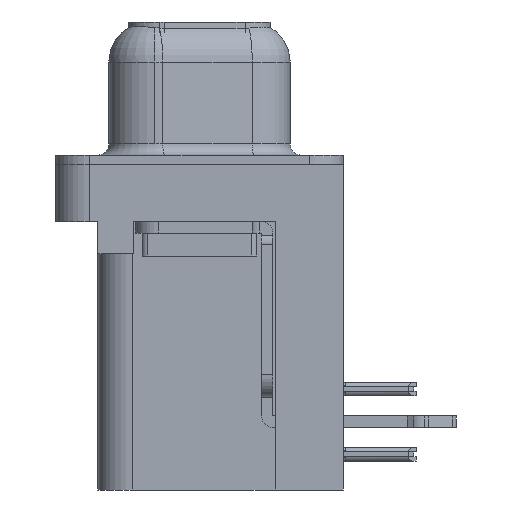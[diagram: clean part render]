
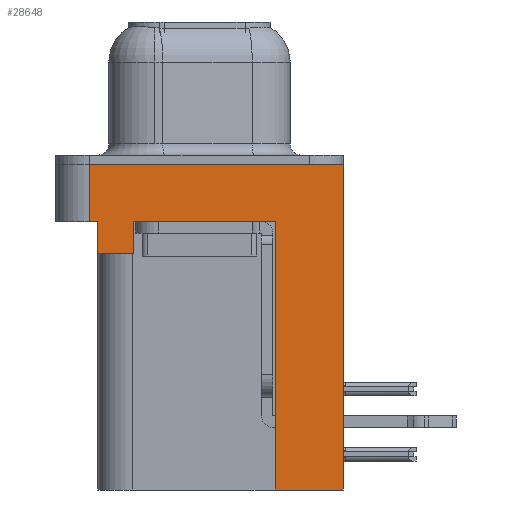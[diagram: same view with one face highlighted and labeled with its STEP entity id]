
A CAD part, left-side view. The second image highlights one B-rep face of the part: STEP entity #28648.
In plain terms, the highlighted planar face has unit normal (-1, 0, 0).
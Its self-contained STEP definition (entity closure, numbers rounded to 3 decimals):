
#189 = CARTESIAN_POINT ( 'NONE',  ( -2.91, 4.425, -3.9 ) ) ;
#225 = EDGE_CURVE ( 'NONE', #4165, #5498, #7820, .T. ) ;
#361 = CARTESIAN_POINT ( 'NONE',  ( -2.91, -6.275, 0. ) ) ;
#401 = LINE ( 'NONE', #21651, #32084 ) ;
#633 = EDGE_CURVE ( 'NONE', #26346, #26637, #401, .T. ) ;
#636 = EDGE_CURVE ( 'NONE', #27054, #9915, #24114, .T. ) ;
#830 = CARTESIAN_POINT ( 'NONE',  ( -2.91, -3.295, -14.2 ) ) ;
#1801 = ORIENTED_EDGE ( 'NONE', *, *, #12141, .F. ) ;
#2073 = CARTESIAN_POINT ( 'NONE',  ( -2.91, 2.895, -2.5 ) ) ;
#3632 = FACE_OUTER_BOUND ( 'NONE', #15709, .T. ) ;
#3735 = CARTESIAN_POINT ( 'NONE',  ( -2.91, 4.775, -2.5 ) ) ;
#4165 = VERTEX_POINT ( 'NONE', #10867 ) ;
#4537 = DIRECTION ( 'NONE',  ( 0., 0., 1. ) ) ;
#4563 = AXIS2_PLACEMENT_3D ( 'NONE', #25066, #22414, #33117 ) ;
#5385 = ORIENTED_EDGE ( 'NONE', *, *, #12654, .F. ) ;
#5498 = VERTEX_POINT ( 'NONE', #2073 ) ;
#5653 = VECTOR ( 'NONE', #29345, 1000. ) ;
#6954 = DIRECTION ( 'NONE',  ( 0., -1., 0. ) ) ;
#7522 = LINE ( 'NONE', #31911, #12522 ) ;
#7767 = VECTOR ( 'NONE', #19387, 1000. ) ;
#7820 = LINE ( 'NONE', #29422, #11222 ) ;
#9086 = VECTOR ( 'NONE', #6954, 1000. ) ;
#9915 = VERTEX_POINT ( 'NONE', #27889 ) ;
#10867 = CARTESIAN_POINT ( 'NONE',  ( -2.91, 2.895, -3.9 ) ) ;
#10979 = DIRECTION ( 'NONE',  ( 0., 0., 1. ) ) ;
#11222 = VECTOR ( 'NONE', #10979, 1000. ) ;
#11522 = EDGE_CURVE ( 'NONE', #5498, #23174, #17658, .T. ) ;
#12141 = EDGE_CURVE ( 'NONE', #19005, #23174, #18481, .T. ) ;
#12441 = CARTESIAN_POINT ( 'NONE',  ( -2.91, -6.275, 0. ) ) ;
#12522 = VECTOR ( 'NONE', #4537, 1000. ) ;
#12654 = EDGE_CURVE ( 'NONE', #26125, #19005, #14173, .T. ) ;
#13568 = VECTOR ( 'NONE', #13749, 1000. ) ;
#13749 = DIRECTION ( 'NONE',  ( 0., 0., 1. ) ) ;
#14173 = LINE ( 'NONE', #830, #22597 ) ;
#14353 = PLANE ( 'NONE',  #4563 ) ;
#15074 = DIRECTION ( 'NONE',  ( 0., 1., 0. ) ) ;
#15709 = EDGE_LOOP ( 'NONE', ( #18794, #30606, #23260, #26864, #33194, #31968, #23399, #1801, #5385, #28310 ) ) ;
#16087 = LINE ( 'NONE', #32043, #7767 ) ;
#17622 = EDGE_CURVE ( 'NONE', #26125, #24102, #7522, .T. ) ;
#17658 = LINE ( 'NONE', #30823, #9086 ) ;
#18481 = LINE ( 'NONE', #29192, #33218 ) ;
#18562 = LINE ( 'NONE', #29279, #31765 ) ;
#18670 = CARTESIAN_POINT ( 'NONE',  ( -2.91, 4.775, -2.5 ) ) ;
#18794 = ORIENTED_EDGE ( 'NONE', *, *, #32624, .F. ) ;
#19005 = VERTEX_POINT ( 'NONE', #27869 ) ;
#19387 = DIRECTION ( 'NONE',  ( 0., -1., 0. ) ) ;
#19695 = CARTESIAN_POINT ( 'NONE',  ( -2.91, -6.275, -14.2 ) ) ;
#19948 = DIRECTION ( 'NONE',  ( 0., 1., 0. ) ) ;
#21651 = CARTESIAN_POINT ( 'NONE',  ( -2.91, 4.425, -3.9 ) ) ;
#22414 = DIRECTION ( 'NONE',  ( -1., 0., 0. ) ) ;
#22597 = VECTOR ( 'NONE', #19948, 1000. ) ;
#23174 = VERTEX_POINT ( 'NONE', #33862 ) ;
#23260 = ORIENTED_EDGE ( 'NONE', *, *, #25615, .T. ) ;
#23273 = EDGE_CURVE ( 'NONE', #4165, #26346, #18562, .T. ) ;
#23399 = ORIENTED_EDGE ( 'NONE', *, *, #11522, .T. ) ;
#23579 = DIRECTION ( 'NONE',  ( 0., 0., 1. ) ) ;
#24102 = VERTEX_POINT ( 'NONE', #12441 ) ;
#24114 = LINE ( 'NONE', #18670, #13568 ) ;
#24418 = LINE ( 'NONE', #361, #5653 ) ;
#25066 = CARTESIAN_POINT ( 'NONE',  ( -2.91, -6.275, -2.5 ) ) ;
#25615 = EDGE_CURVE ( 'NONE', #27054, #26637, #16087, .T. ) ;
#26125 = VERTEX_POINT ( 'NONE', #19695 ) ;
#26346 = VERTEX_POINT ( 'NONE', #189 ) ;
#26637 = VERTEX_POINT ( 'NONE', #27352 ) ;
#26751 = DIRECTION ( 'NONE',  ( 0., 0., 1. ) ) ;
#26864 = ORIENTED_EDGE ( 'NONE', *, *, #633, .F. ) ;
#27054 = VERTEX_POINT ( 'NONE', #3735 ) ;
#27352 = CARTESIAN_POINT ( 'NONE',  ( -2.91, 4.425, -2.5 ) ) ;
#27869 = CARTESIAN_POINT ( 'NONE',  ( -2.91, -3.295, -14.2 ) ) ;
#27889 = CARTESIAN_POINT ( 'NONE',  ( -2.91, 4.775, 0. ) ) ;
#28310 = ORIENTED_EDGE ( 'NONE', *, *, #17622, .T. ) ;
#28648 = ADVANCED_FACE ( 'NONE', ( #3632 ), #14353, .T. ) ;
#29192 = CARTESIAN_POINT ( 'NONE',  ( -2.91, -3.295, -14.2 ) ) ;
#29279 = CARTESIAN_POINT ( 'NONE',  ( -2.91, 4.425, -3.9 ) ) ;
#29345 = DIRECTION ( 'NONE',  ( 0., -1., 0. ) ) ;
#29422 = CARTESIAN_POINT ( 'NONE',  ( -2.91, 2.895, -3.9 ) ) ;
#30606 = ORIENTED_EDGE ( 'NONE', *, *, #636, .F. ) ;
#30823 = CARTESIAN_POINT ( 'NONE',  ( -2.91, -6.275, -2.5 ) ) ;
#31765 = VECTOR ( 'NONE', #15074, 1000. ) ;
#31911 = CARTESIAN_POINT ( 'NONE',  ( -2.91, -6.275, -2.5 ) ) ;
#31968 = ORIENTED_EDGE ( 'NONE', *, *, #225, .T. ) ;
#32043 = CARTESIAN_POINT ( 'NONE',  ( -2.91, -6.275, -2.5 ) ) ;
#32084 = VECTOR ( 'NONE', #26751, 1000. ) ;
#32624 = EDGE_CURVE ( 'NONE', #9915, #24102, #24418, .T. ) ;
#33117 = DIRECTION ( 'NONE',  ( 0., 0., 1. ) ) ;
#33194 = ORIENTED_EDGE ( 'NONE', *, *, #23273, .F. ) ;
#33218 = VECTOR ( 'NONE', #23579, 1000. ) ;
#33862 = CARTESIAN_POINT ( 'NONE',  ( -2.91, -3.295, -2.5 ) ) ;
